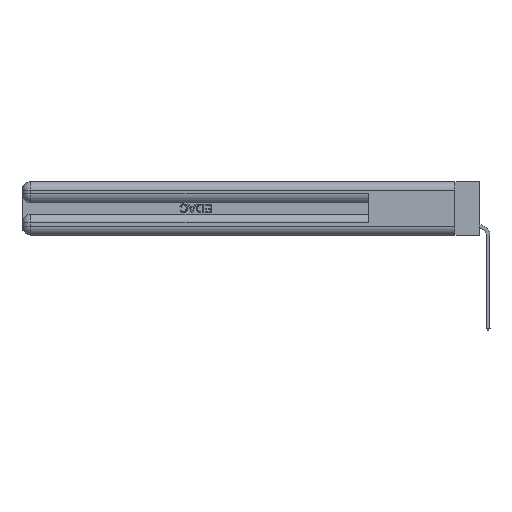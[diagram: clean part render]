
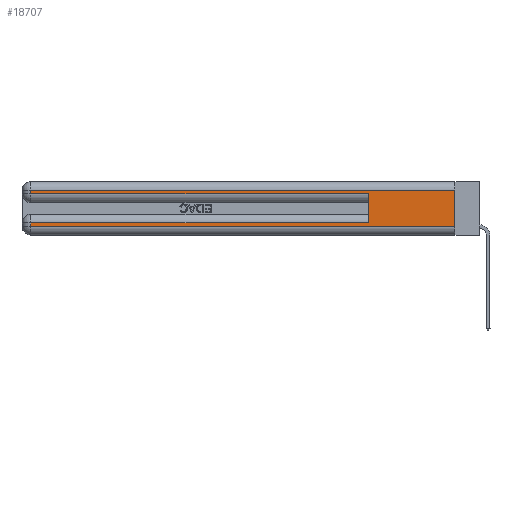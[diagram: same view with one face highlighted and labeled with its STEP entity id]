
A CAD part, left-side view. The second image highlights one B-rep face of the part: STEP entity #18707.
In plain terms, the highlighted planar face has unit normal (-1, 0, 0).
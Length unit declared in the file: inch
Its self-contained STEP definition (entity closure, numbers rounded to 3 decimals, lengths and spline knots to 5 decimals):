
#243 = CARTESIAN_POINT ( 'NONE',  ( 0., 2.94, 0.085 ) ) ;
#1126 = DIRECTION ( 'NONE',  ( 0., -1., 0. ) ) ;
#1269 = LINE ( 'NONE', #1566, #11548 ) ;
#1361 = VERTEX_POINT ( 'NONE', #243 ) ;
#1566 = CARTESIAN_POINT ( 'NONE',  ( 0., 2.94, 0.37 ) ) ;
#1702 = VERTEX_POINT ( 'NONE', #16011 ) ;
#1819 = VERTEX_POINT ( 'NONE', #16323 ) ;
#4273 = LINE ( 'NONE', #30566, #8266 ) ;
#4580 = DIRECTION ( 'NONE',  ( 0., 0., -1. ) ) ;
#4642 = VERTEX_POINT ( 'NONE', #17456 ) ;
#4700 = DIRECTION ( 'NONE',  ( 0., 1., 0. ) ) ;
#5448 = CARTESIAN_POINT ( 'NONE',  ( 0., 0., 0.37 ) ) ;
#5466 = ORIENTED_EDGE ( 'NONE', *, *, #22832, .T. ) ;
#5697 = ORIENTED_EDGE ( 'NONE', *, *, #29020, .T. ) ;
#5984 = CARTESIAN_POINT ( 'NONE',  ( 0., 0.6, 0.145 ) ) ;
#6283 = VECTOR ( 'NONE', #1126, 39.37008 ) ;
#6762 = DIRECTION ( 'NONE',  ( 0., 0., -1. ) ) ;
#7396 = EDGE_CURVE ( 'NONE', #1702, #25149, #4273, .T. ) ;
#8266 = VECTOR ( 'NONE', #4580, 39.37008 ) ;
#8473 = ORIENTED_EDGE ( 'NONE', *, *, #12648, .T. ) ;
#10103 = ORIENTED_EDGE ( 'NONE', *, *, #17845, .F. ) ;
#10186 = LINE ( 'NONE', #22090, #26830 ) ;
#10766 = DIRECTION ( 'NONE',  ( 0., 1., 0. ) ) ;
#11101 = DIRECTION ( 'NONE',  ( 0., 0., -1. ) ) ;
#11548 = VECTOR ( 'NONE', #11101, 39.37008 ) ;
#11593 = VERTEX_POINT ( 'NONE', #18885 ) ;
#12444 = CARTESIAN_POINT ( 'NONE',  ( 0., 0., 0.285 ) ) ;
#12648 = EDGE_CURVE ( 'NONE', #11593, #25149, #27727, .T. ) ;
#12826 = ORIENTED_EDGE ( 'NONE', *, *, #25910, .T. ) ;
#12953 = CARTESIAN_POINT ( 'NONE',  ( 0., 0., 0.085 ) ) ;
#13090 = DIRECTION ( 'NONE',  ( 0., 0., -1. ) ) ;
#13313 = CARTESIAN_POINT ( 'NONE',  ( 0., 0., 0.06 ) ) ;
#14098 = VECTOR ( 'NONE', #19631, 39.37008 ) ;
#15424 = DIRECTION ( 'NONE',  ( 0., -1., 0. ) ) ;
#16011 = CARTESIAN_POINT ( 'NONE',  ( 0., 0., 0.31 ) ) ;
#16262 = VECTOR ( 'NONE', #6762, 39.37008 ) ;
#16323 = CARTESIAN_POINT ( 'NONE',  ( 0., 0.6, 0.085 ) ) ;
#16643 = AXIS2_PLACEMENT_3D ( 'NONE', #5448, #22665, #13090 ) ;
#17337 = FACE_OUTER_BOUND ( 'NONE', #22888, .T. ) ;
#17456 = CARTESIAN_POINT ( 'NONE',  ( 0., 2.94, 0.285 ) ) ;
#17494 = PLANE ( 'NONE',  #16643 ) ;
#17665 = LINE ( 'NONE', #12953, #25572 ) ;
#17728 = VECTOR ( 'NONE', #15424, 39.37008 ) ;
#17845 = EDGE_CURVE ( 'NONE', #1819, #22455, #17871, .T. ) ;
#17871 = LINE ( 'NONE', #5984, #14098 ) ;
#18707 = ADVANCED_FACE ( 'NONE', ( #17337 ), #17494, .F. ) ;
#18885 = CARTESIAN_POINT ( 'NONE',  ( 0., 2.94, 0.06 ) ) ;
#19631 = DIRECTION ( 'NONE',  ( 0., 0., 1. ) ) ;
#21974 = CARTESIAN_POINT ( 'NONE',  ( 0., 0.6, 0.285 ) ) ;
#22090 = CARTESIAN_POINT ( 'NONE',  ( 0., 0., 0.31 ) ) ;
#22100 = EDGE_CURVE ( 'NONE', #4642, #22455, #24843, .T. ) ;
#22455 = VERTEX_POINT ( 'NONE', #21974 ) ;
#22665 = DIRECTION ( 'NONE',  ( 1., 0., 0. ) ) ;
#22832 = EDGE_CURVE ( 'NONE', #24579, #4642, #26010, .T. ) ;
#22888 = EDGE_LOOP ( 'NONE', ( #26997, #12826, #5466, #27571, #10103, #5697, #26486, #8473 ) ) ;
#24579 = VERTEX_POINT ( 'NONE', #30663 ) ;
#24843 = LINE ( 'NONE', #12444, #17728 ) ;
#25149 = VERTEX_POINT ( 'NONE', #26408 ) ;
#25572 = VECTOR ( 'NONE', #10766, 39.37008 ) ;
#25910 = EDGE_CURVE ( 'NONE', #1702, #24579, #10186, .T. ) ;
#26010 = LINE ( 'NONE', #28047, #16262 ) ;
#26408 = CARTESIAN_POINT ( 'NONE',  ( 0., 0., 0.06 ) ) ;
#26486 = ORIENTED_EDGE ( 'NONE', *, *, #28725, .T. ) ;
#26830 = VECTOR ( 'NONE', #4700, 39.37008 ) ;
#26997 = ORIENTED_EDGE ( 'NONE', *, *, #7396, .F. ) ;
#27571 = ORIENTED_EDGE ( 'NONE', *, *, #22100, .T. ) ;
#27727 = LINE ( 'NONE', #13313, #6283 ) ;
#28047 = CARTESIAN_POINT ( 'NONE',  ( 0., 2.94, 0.37 ) ) ;
#28725 = EDGE_CURVE ( 'NONE', #1361, #11593, #1269, .T. ) ;
#29020 = EDGE_CURVE ( 'NONE', #1819, #1361, #17665, .T. ) ;
#30566 = CARTESIAN_POINT ( 'NONE',  ( 0., 0., 0.37 ) ) ;
#30663 = CARTESIAN_POINT ( 'NONE',  ( 0., 2.94, 0.31 ) ) ;
